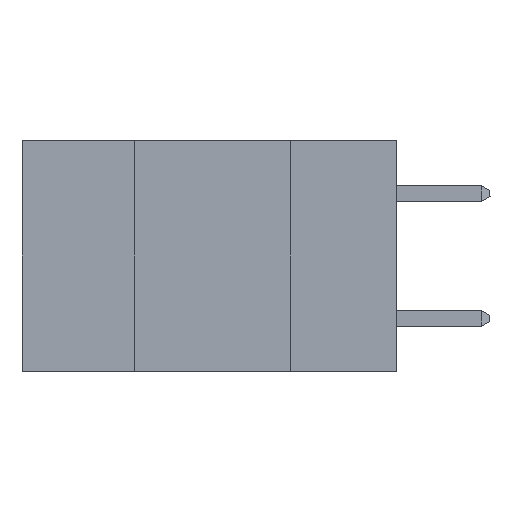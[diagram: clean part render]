
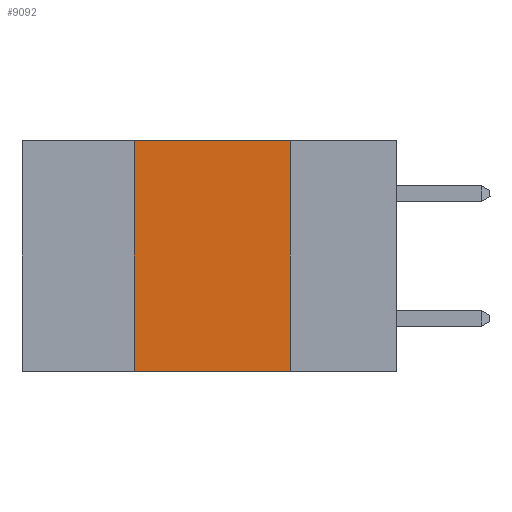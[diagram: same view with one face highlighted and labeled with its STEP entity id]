
A CAD part, left-side view. The second image highlights one B-rep face of the part: STEP entity #9092.
In plain terms, the highlighted planar face has unit normal (-1, 0, 0).
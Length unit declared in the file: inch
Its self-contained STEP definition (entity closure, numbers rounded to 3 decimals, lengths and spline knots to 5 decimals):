
#249 = CARTESIAN_POINT ( 'NONE',  ( 0., 0.17, 0. ) ) ;
#863 = VERTEX_POINT ( 'NONE', #5068 ) ;
#971 = VECTOR ( 'NONE', #17725, 39.37008 ) ;
#1318 = VERTEX_POINT ( 'NONE', #13748 ) ;
#1488 = PLANE ( 'NONE',  #6966 ) ;
#1552 = CARTESIAN_POINT ( 'NONE',  ( 0., 0.6, 0. ) ) ;
#1557 = DIRECTION ( 'NONE',  ( 0., 0., -1. ) ) ;
#1612 = DIRECTION ( 'NONE',  ( 1., 0., 0. ) ) ;
#2229 = EDGE_CURVE ( 'NONE', #1318, #14406, #4794, .T. ) ;
#2434 = CARTESIAN_POINT ( 'NONE',  ( 0., 0.42, 0. ) ) ;
#3394 = EDGE_CURVE ( 'NONE', #7546, #863, #14704, .T. ) ;
#3830 = EDGE_CURVE ( 'NONE', #14406, #7546, #14824, .T. ) ;
#4072 = VECTOR ( 'NONE', #1557, 39.37008 ) ;
#4291 = CARTESIAN_POINT ( 'NONE',  ( 0., 0.6, 0. ) ) ;
#4794 = LINE ( 'NONE', #2434, #8439 ) ;
#5068 = CARTESIAN_POINT ( 'NONE',  ( 0., 0.17, -0.37 ) ) ;
#5576 = CARTESIAN_POINT ( 'NONE',  ( 0., 0.6, -0.37 ) ) ;
#6055 = ORIENTED_EDGE ( 'NONE', *, *, #3830, .F. ) ;
#6532 = LINE ( 'NONE', #5576, #11510 ) ;
#6966 = AXIS2_PLACEMENT_3D ( 'NONE', #4291, #1612, #8568 ) ;
#7546 = VERTEX_POINT ( 'NONE', #17703 ) ;
#8439 = VECTOR ( 'NONE', #16181, 39.37008 ) ;
#8568 = DIRECTION ( 'NONE',  ( 0., 0., -1. ) ) ;
#9092 = ADVANCED_FACE ( 'NONE', ( #10953 ), #1488, .F. ) ;
#9519 = ORIENTED_EDGE ( 'NONE', *, *, #2229, .F. ) ;
#10788 = CARTESIAN_POINT ( 'NONE',  ( 0., 0.42, 0. ) ) ;
#10953 = FACE_OUTER_BOUND ( 'NONE', #16580, .T. ) ;
#11510 = VECTOR ( 'NONE', #16773, 39.37008 ) ;
#11848 = ORIENTED_EDGE ( 'NONE', *, *, #3394, .F. ) ;
#13748 = CARTESIAN_POINT ( 'NONE',  ( 0., 0.42, -0.37 ) ) ;
#14406 = VERTEX_POINT ( 'NONE', #10788 ) ;
#14455 = EDGE_CURVE ( 'NONE', #1318, #863, #6532, .T. ) ;
#14534 = ORIENTED_EDGE ( 'NONE', *, *, #14455, .T. ) ;
#14704 = LINE ( 'NONE', #249, #4072 ) ;
#14824 = LINE ( 'NONE', #1552, #971 ) ;
#16181 = DIRECTION ( 'NONE',  ( 0., 0., 1. ) ) ;
#16580 = EDGE_LOOP ( 'NONE', ( #11848, #6055, #9519, #14534 ) ) ;
#16773 = DIRECTION ( 'NONE',  ( 0., -1., 0. ) ) ;
#17703 = CARTESIAN_POINT ( 'NONE',  ( 0., 0.17, 0. ) ) ;
#17725 = DIRECTION ( 'NONE',  ( 0., -1., 0. ) ) ;
